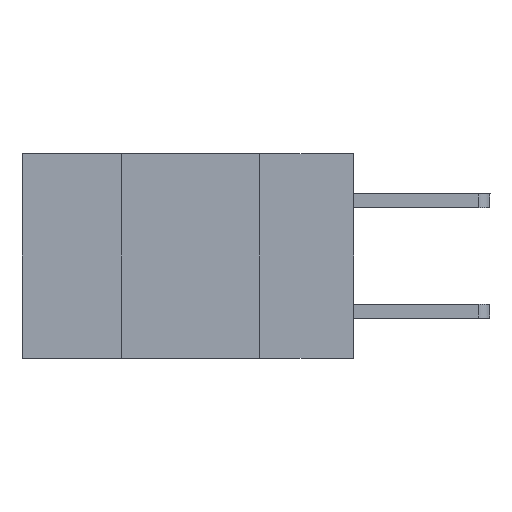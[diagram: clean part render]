
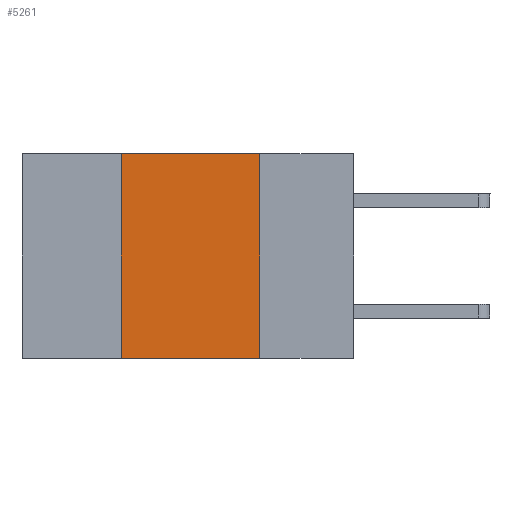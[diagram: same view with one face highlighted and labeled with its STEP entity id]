
A CAD part, left-side view. The second image highlights one B-rep face of the part: STEP entity #5261.
In plain terms, the highlighted planar face has unit normal (-1, 0, 0).
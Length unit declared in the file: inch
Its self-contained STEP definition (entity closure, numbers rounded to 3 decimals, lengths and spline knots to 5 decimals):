
#475 = CARTESIAN_POINT ( 'NONE',  ( 0., 0.42, 0. ) ) ;
#1548 = DIRECTION ( 'NONE',  ( 1., 0., 0. ) ) ;
#2031 = EDGE_CURVE ( 'NONE', #9394, #3237, #5911, .T. ) ;
#2135 = CARTESIAN_POINT ( 'NONE',  ( 0., 0.42, 0. ) ) ;
#2398 = VERTEX_POINT ( 'NONE', #5350 ) ;
#2905 = VECTOR ( 'NONE', #3207, 39.37008 ) ;
#3207 = DIRECTION ( 'NONE',  ( 0., 0., 1. ) ) ;
#3237 = VERTEX_POINT ( 'NONE', #8731 ) ;
#3243 = LINE ( 'NONE', #6281, #6239 ) ;
#3843 = LINE ( 'NONE', #8109, #6844 ) ;
#3960 = CARTESIAN_POINT ( 'NONE',  ( 0., 0.6, 0. ) ) ;
#4418 = FACE_OUTER_BOUND ( 'NONE', #5973, .T. ) ;
#4586 = ORIENTED_EDGE ( 'NONE', *, *, #6055, .F. ) ;
#4600 = DIRECTION ( 'NONE',  ( 0., -1., 0. ) ) ;
#4706 = ORIENTED_EDGE ( 'NONE', *, *, #2031, .F. ) ;
#4905 = ORIENTED_EDGE ( 'NONE', *, *, #9003, .T. ) ;
#5261 = ADVANCED_FACE ( 'NONE', ( #4418 ), #10605, .F. ) ;
#5350 = CARTESIAN_POINT ( 'NONE',  ( 0., 0.42, -0.37 ) ) ;
#5503 = CARTESIAN_POINT ( 'NONE',  ( 0., 0.17, 0. ) ) ;
#5911 = LINE ( 'NONE', #5503, #7734 ) ;
#5973 = EDGE_LOOP ( 'NONE', ( #4706, #4586, #8570, #4905 ) ) ;
#6055 = EDGE_CURVE ( 'NONE', #6071, #9394, #3243, .T. ) ;
#6071 = VERTEX_POINT ( 'NONE', #2135 ) ;
#6239 = VECTOR ( 'NONE', #9617, 39.37008 ) ;
#6281 = CARTESIAN_POINT ( 'NONE',  ( 0., 0.6, 0. ) ) ;
#6452 = DIRECTION ( 'NONE',  ( 0., 0., -1. ) ) ;
#6844 = VECTOR ( 'NONE', #4600, 39.37008 ) ;
#7734 = VECTOR ( 'NONE', #6452, 39.37008 ) ;
#8109 = CARTESIAN_POINT ( 'NONE',  ( 0., 0.6, -0.37 ) ) ;
#8137 = LINE ( 'NONE', #475, #2905 ) ;
#8222 = AXIS2_PLACEMENT_3D ( 'NONE', #3960, #1548, #10755 ) ;
#8570 = ORIENTED_EDGE ( 'NONE', *, *, #10571, .F. ) ;
#8731 = CARTESIAN_POINT ( 'NONE',  ( 0., 0.17, -0.37 ) ) ;
#9003 = EDGE_CURVE ( 'NONE', #2398, #3237, #3843, .T. ) ;
#9083 = CARTESIAN_POINT ( 'NONE',  ( 0., 0.17, 0. ) ) ;
#9394 = VERTEX_POINT ( 'NONE', #9083 ) ;
#9617 = DIRECTION ( 'NONE',  ( 0., -1., 0. ) ) ;
#10571 = EDGE_CURVE ( 'NONE', #2398, #6071, #8137, .T. ) ;
#10605 = PLANE ( 'NONE',  #8222 ) ;
#10755 = DIRECTION ( 'NONE',  ( 0., 0., -1. ) ) ;
